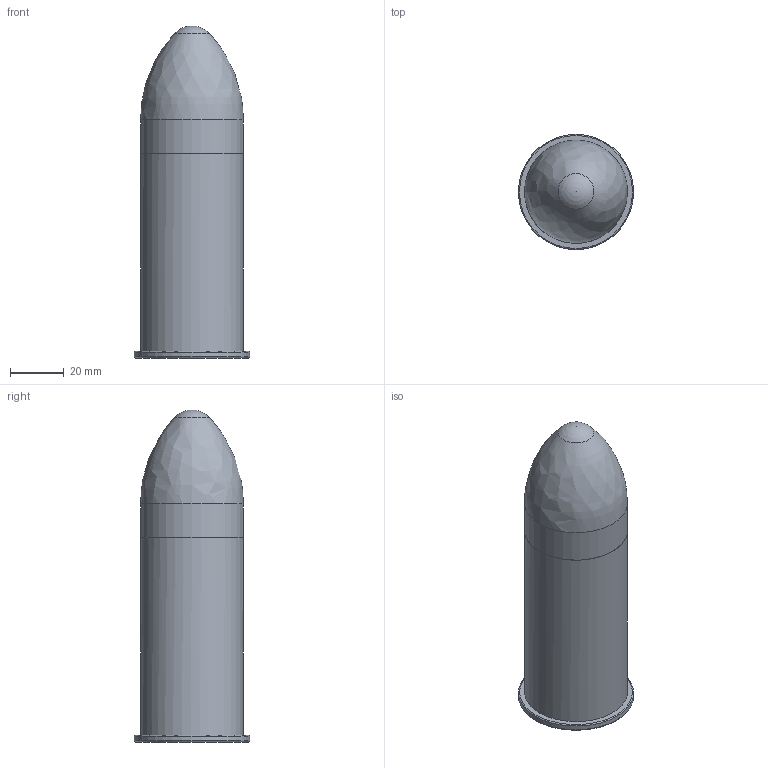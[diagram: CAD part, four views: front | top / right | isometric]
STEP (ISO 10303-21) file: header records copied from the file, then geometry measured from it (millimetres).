
FILE_DESCRIPTION(/* description */ (''),/* implementation_level */ '2;1');
FILE_NAME(/* name */ 'Threaded 3in Casing BETA.step',/* time_stamp */ '2021-09-02T02:11:28-04:00',/* author */ (''),/* organization */ (''),/* preprocessor_version */ 'ST-DEVELOPER v18.1',/* originating_system */ 'Autodesk Translation Framework v10.10.0.1391',/* authorisation */ '');
FILE_SCHEMA (('AUTOMOTIVE_DESIGN { 1 0 10303 214 3 1 1 }'));
Length unit declared in the file: millimetre
Products named in the file (1): Threaded 3in Casing
Bounding box: 42.93 x 42.93 x 123.7 mm (x, y, z)
Volume: 76633.4 mm3; surface area: 47357.3 mm2
Topology: 4 solids, 4 shells, 101 faces, 264 edges, 173 vertices
Faces by surface type: cylinder 47, bspline 26, plane 10, torus 9, cone 7, sphere 2
Full cylindrical faces by diameter (mm): 6.3 x1, 8.8 x1, 9 x1, 25.254 x1, 25.754 x1, 26.33 x7, 27.002 x7, 29.415 x7, 30.349 x7, 33.754 x1, 34.354 x1, 34.854 x1, 38.354 x2, 42.93 x1
Entity records: 8451 total; most frequent: CARTESIAN_POINT 6170, ORIENTED_EDGE 524, DIRECTION 360, EDGE_CURVE 262, VERTEX_POINT 173, AXIS2_PLACEMENT_3D 145, B_SPLINE_CURVE_WITH_KNOTS 123, EDGE_LOOP 109
